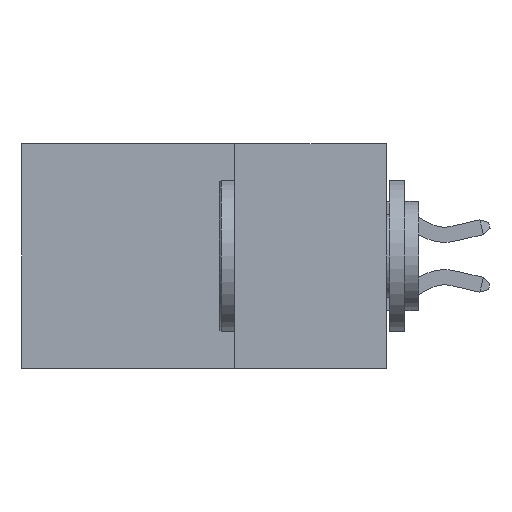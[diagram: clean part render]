
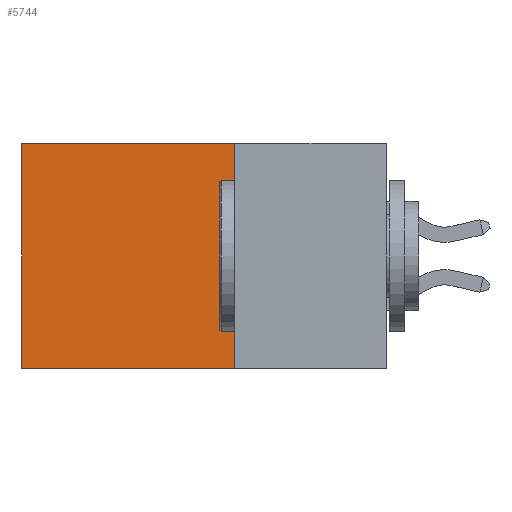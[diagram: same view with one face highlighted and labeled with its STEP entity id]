
A CAD part, left-side view. The second image highlights one B-rep face of the part: STEP entity #5744.
In plain terms, the highlighted planar face has unit normal (-1, 0, 0).
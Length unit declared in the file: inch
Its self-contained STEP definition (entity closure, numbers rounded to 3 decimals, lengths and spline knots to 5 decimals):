
#341 = LINE ( 'NONE', #18513, #11195 ) ;
#743 = CARTESIAN_POINT ( 'NONE',  ( 0.298, 0.25, -0.37 ) ) ;
#886 = DIRECTION ( 'NONE',  ( 0., 1., 0. ) ) ;
#2329 = EDGE_CURVE ( 'NONE', #5276, #15787, #2613, .T. ) ;
#2460 = CARTESIAN_POINT ( 'NONE',  ( 0.298, 0.6, -0.37 ) ) ;
#2613 = LINE ( 'NONE', #16246, #13638 ) ;
#2661 = FACE_OUTER_BOUND ( 'NONE', #4374, .T. ) ;
#3275 = VECTOR ( 'NONE', #6611, 39.37008 ) ;
#4374 = EDGE_LOOP ( 'NONE', ( #13131, #8702, #14962, #4697 ) ) ;
#4676 = LINE ( 'NONE', #7147, #11826 ) ;
#4697 = ORIENTED_EDGE ( 'NONE', *, *, #5435, .T. ) ;
#5276 = VERTEX_POINT ( 'NONE', #10333 ) ;
#5435 = EDGE_CURVE ( 'NONE', #10261, #5276, #4676, .T. ) ;
#5732 = CARTESIAN_POINT ( 'NONE',  ( 0.298, 0.25, -0.37 ) ) ;
#5744 = ADVANCED_FACE ( 'NONE', ( #2661 ), #14289, .F. ) ;
#6611 = DIRECTION ( 'NONE',  ( 0., 1., 0. ) ) ;
#7068 = EDGE_CURVE ( 'NONE', #10454, #15787, #14815, .T. ) ;
#7147 = CARTESIAN_POINT ( 'NONE',  ( 0.298, 0.25, 0. ) ) ;
#8702 = ORIENTED_EDGE ( 'NONE', *, *, #7068, .F. ) ;
#10035 = DIRECTION ( 'NONE',  ( 0., 0., -1. ) ) ;
#10261 = VERTEX_POINT ( 'NONE', #13184 ) ;
#10333 = CARTESIAN_POINT ( 'NONE',  ( 0.298, 0.6, 0. ) ) ;
#10454 = VERTEX_POINT ( 'NONE', #743 ) ;
#11195 = VECTOR ( 'NONE', #12673, 39.37008 ) ;
#11826 = VECTOR ( 'NONE', #886, 39.37008 ) ;
#11974 = EDGE_CURVE ( 'NONE', #10261, #10454, #341, .T. ) ;
#12502 = DIRECTION ( 'NONE',  ( 1., 0., 0. ) ) ;
#12673 = DIRECTION ( 'NONE',  ( 0., 0., -1. ) ) ;
#12940 = DIRECTION ( 'NONE',  ( 0., 0., -1. ) ) ;
#13131 = ORIENTED_EDGE ( 'NONE', *, *, #2329, .T. ) ;
#13184 = CARTESIAN_POINT ( 'NONE',  ( 0.298, 0.25, 0. ) ) ;
#13403 = CARTESIAN_POINT ( 'NONE',  ( 0.298, 0.25, 0. ) ) ;
#13455 = AXIS2_PLACEMENT_3D ( 'NONE', #13403, #12502, #12940 ) ;
#13638 = VECTOR ( 'NONE', #10035, 39.37008 ) ;
#14289 = PLANE ( 'NONE',  #13455 ) ;
#14815 = LINE ( 'NONE', #5732, #3275 ) ;
#14962 = ORIENTED_EDGE ( 'NONE', *, *, #11974, .F. ) ;
#15787 = VERTEX_POINT ( 'NONE', #2460 ) ;
#16246 = CARTESIAN_POINT ( 'NONE',  ( 0.298, 0.6, 0. ) ) ;
#18513 = CARTESIAN_POINT ( 'NONE',  ( 0.298, 0.25, 0. ) ) ;
